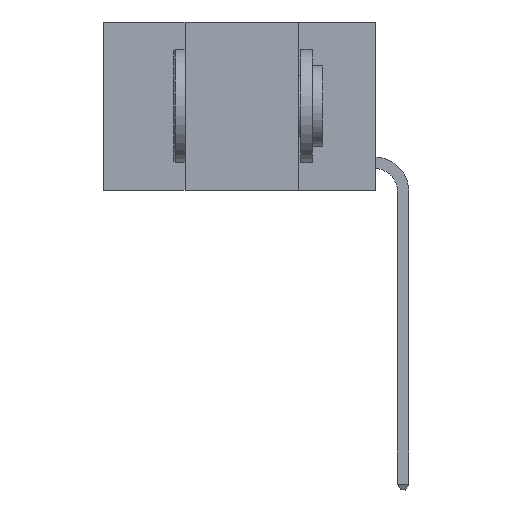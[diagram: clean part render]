
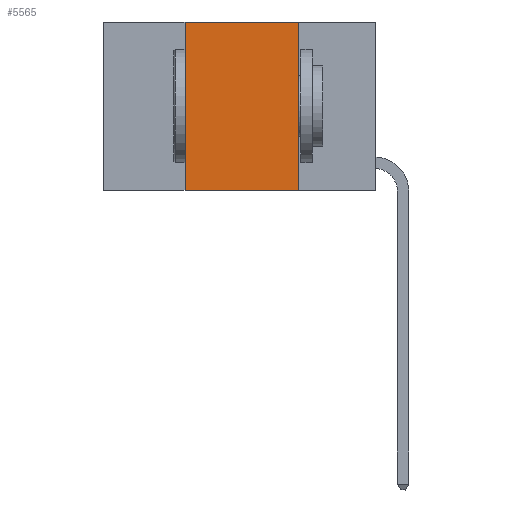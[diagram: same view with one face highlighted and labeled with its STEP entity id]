
A CAD part, left-side view. The second image highlights one B-rep face of the part: STEP entity #5565.
In plain terms, the highlighted planar face has unit normal (-1, 0, 0).
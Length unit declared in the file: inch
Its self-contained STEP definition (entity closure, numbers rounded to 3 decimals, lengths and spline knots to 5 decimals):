
#187 = CARTESIAN_POINT ( 'NONE',  ( 0., 0.6, 0. ) ) ;
#656 = CARTESIAN_POINT ( 'NONE',  ( 0., 0.6, -0.37 ) ) ;
#1902 = CARTESIAN_POINT ( 'NONE',  ( 0., 0.42, 0. ) ) ;
#2117 = DIRECTION ( 'NONE',  ( 0., -1., 0. ) ) ;
#2281 = VERTEX_POINT ( 'NONE', #13560 ) ;
#3169 = EDGE_CURVE ( 'NONE', #8078, #7709, #12057, .T. ) ;
#3718 = VERTEX_POINT ( 'NONE', #5487 ) ;
#3949 = AXIS2_PLACEMENT_3D ( 'NONE', #10971, #6963, #16135 ) ;
#4480 = CARTESIAN_POINT ( 'NONE',  ( 0., 0.42, 0. ) ) ;
#4903 = VECTOR ( 'NONE', #16672, 39.37008 ) ;
#5487 = CARTESIAN_POINT ( 'NONE',  ( 0., 0.17, 0. ) ) ;
#5565 = ADVANCED_FACE ( 'NONE', ( #7614 ), #12349, .F. ) ;
#5672 = VECTOR ( 'NONE', #2117, 39.37008 ) ;
#6121 = LINE ( 'NONE', #656, #5672 ) ;
#6963 = DIRECTION ( 'NONE',  ( 1., 0., 0. ) ) ;
#7336 = ORIENTED_EDGE ( 'NONE', *, *, #9159, .F. ) ;
#7614 = FACE_OUTER_BOUND ( 'NONE', #12798, .T. ) ;
#7709 = VERTEX_POINT ( 'NONE', #4480 ) ;
#7871 = EDGE_CURVE ( 'NONE', #8078, #2281, #6121, .T. ) ;
#8078 = VERTEX_POINT ( 'NONE', #10010 ) ;
#8390 = CARTESIAN_POINT ( 'NONE',  ( 0., 0.17, 0. ) ) ;
#9113 = LINE ( 'NONE', #8390, #15569 ) ;
#9159 = EDGE_CURVE ( 'NONE', #7709, #3718, #15640, .T. ) ;
#9736 = DIRECTION ( 'NONE',  ( 0., 0., -1. ) ) ;
#10010 = CARTESIAN_POINT ( 'NONE',  ( 0., 0.42, -0.37 ) ) ;
#10506 = ORIENTED_EDGE ( 'NONE', *, *, #14300, .F. ) ;
#10579 = DIRECTION ( 'NONE',  ( 0., 0., 1. ) ) ;
#10971 = CARTESIAN_POINT ( 'NONE',  ( 0., 0.6, 0. ) ) ;
#11387 = ORIENTED_EDGE ( 'NONE', *, *, #7871, .T. ) ;
#12057 = LINE ( 'NONE', #1902, #12456 ) ;
#12349 = PLANE ( 'NONE',  #3949 ) ;
#12456 = VECTOR ( 'NONE', #10579, 39.37008 ) ;
#12798 = EDGE_LOOP ( 'NONE', ( #10506, #7336, #14367, #11387 ) ) ;
#13560 = CARTESIAN_POINT ( 'NONE',  ( 0., 0.17, -0.37 ) ) ;
#14300 = EDGE_CURVE ( 'NONE', #3718, #2281, #9113, .T. ) ;
#14367 = ORIENTED_EDGE ( 'NONE', *, *, #3169, .F. ) ;
#15569 = VECTOR ( 'NONE', #9736, 39.37008 ) ;
#15640 = LINE ( 'NONE', #187, #4903 ) ;
#16135 = DIRECTION ( 'NONE',  ( 0., 0., -1. ) ) ;
#16672 = DIRECTION ( 'NONE',  ( 0., -1., 0. ) ) ;
